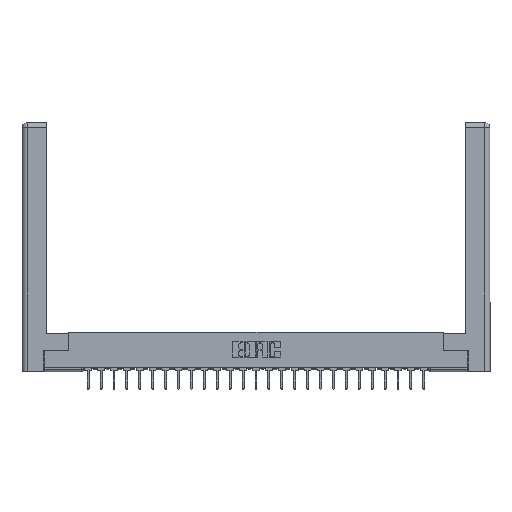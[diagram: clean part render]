
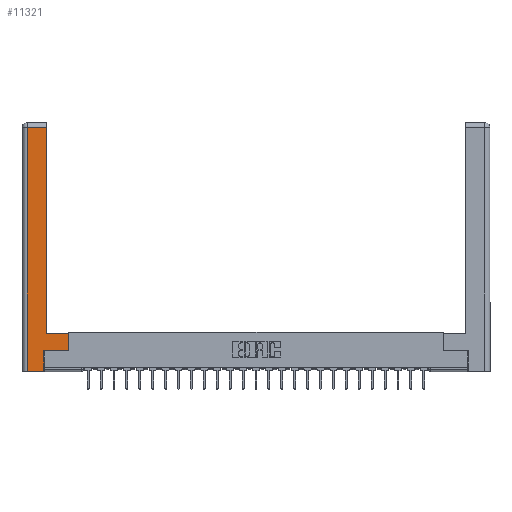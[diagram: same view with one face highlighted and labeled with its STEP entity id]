
A CAD part, top view. The second image highlights one B-rep face of the part: STEP entity #11321.
In plain terms, the highlighted planar face has unit normal (0, 0, 1).
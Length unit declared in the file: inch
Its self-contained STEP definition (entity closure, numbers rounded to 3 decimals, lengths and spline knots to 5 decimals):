
#91 = DIRECTION ( 'NONE',  ( 0., 1., 0. ) ) ;
#453 = VERTEX_POINT ( 'NONE', #3930 ) ;
#1445 = DIRECTION ( 'NONE',  ( 0., -1., 0. ) ) ;
#2126 = LINE ( 'NONE', #8370, #24151 ) ;
#2613 = VERTEX_POINT ( 'NONE', #10627 ) ;
#3254 = LINE ( 'NONE', #16500, #15256 ) ;
#3927 = LINE ( 'NONE', #7426, #9118 ) ;
#3930 = CARTESIAN_POINT ( 'NONE',  ( 0.565, 0.45, 0. ) ) ;
#4493 = VECTOR ( 'NONE', #9994, 39.37008 ) ;
#4917 = VERTEX_POINT ( 'NONE', #18198 ) ;
#4936 = FACE_OUTER_BOUND ( 'NONE', #17056, .T. ) ;
#4979 = VECTOR ( 'NONE', #1445, 39.37008 ) ;
#6336 = DIRECTION ( 'NONE',  ( 0., 1., 0. ) ) ;
#7166 = ORIENTED_EDGE ( 'NONE', *, *, #22486, .T. ) ;
#7337 = CARTESIAN_POINT ( 'NONE',  ( 0.295, 0.45, 0. ) ) ;
#7426 = CARTESIAN_POINT ( 'NONE',  ( 0.565, 0.45, 0. ) ) ;
#7503 = VERTEX_POINT ( 'NONE', #7896 ) ;
#7896 = CARTESIAN_POINT ( 'NONE',  ( 0.265, 0.245, 0. ) ) ;
#8370 = CARTESIAN_POINT ( 'NONE',  ( 0.265, 0.245, 0. ) ) ;
#8605 = VERTEX_POINT ( 'NONE', #7337 ) ;
#9118 = VECTOR ( 'NONE', #16224, 39.37008 ) ;
#9213 = CARTESIAN_POINT ( 'NONE',  ( 0.0615, 2.94, 0. ) ) ;
#9342 = LINE ( 'NONE', #14629, #14463 ) ;
#9994 = DIRECTION ( 'NONE',  ( -1., 0., 0. ) ) ;
#10014 = DIRECTION ( 'NONE',  ( 1., 0., 0. ) ) ;
#10089 = AXIS2_PLACEMENT_3D ( 'NONE', #15888, #20520, #24649 ) ;
#10627 = CARTESIAN_POINT ( 'NONE',  ( 0.565, 0.245, 0. ) ) ;
#10647 = EDGE_CURVE ( 'NONE', #2613, #453, #3927, .T. ) ;
#10920 = VERTEX_POINT ( 'NONE', #11051 ) ;
#11051 = CARTESIAN_POINT ( 'NONE',  ( 0.265, 0., 0. ) ) ;
#11321 = ADVANCED_FACE ( 'NONE', ( #4936 ), #16072, .F. ) ;
#12737 = LINE ( 'NONE', #27295, #4493 ) ;
#13498 = DIRECTION ( 'NONE',  ( -1., 0., 0. ) ) ;
#14463 = VECTOR ( 'NONE', #91, 39.37008 ) ;
#14501 = CARTESIAN_POINT ( 'NONE',  ( 0.0615, 0., 0. ) ) ;
#14629 = CARTESIAN_POINT ( 'NONE',  ( 0.295, 3., 0. ) ) ;
#14722 = EDGE_CURVE ( 'NONE', #7503, #2613, #15604, .T. ) ;
#15256 = VECTOR ( 'NONE', #10014, 39.37008 ) ;
#15604 = LINE ( 'NONE', #20770, #19044 ) ;
#15867 = CARTESIAN_POINT ( 'NONE',  ( 0.0615, 2.94, 0. ) ) ;
#15888 = CARTESIAN_POINT ( 'NONE',  ( 0., 0., 0. ) ) ;
#16072 = PLANE ( 'NONE',  #10089 ) ;
#16224 = DIRECTION ( 'NONE',  ( 0., 1., 0. ) ) ;
#16500 = CARTESIAN_POINT ( 'NONE',  ( 0.265, 0., 0. ) ) ;
#16535 = ORIENTED_EDGE ( 'NONE', *, *, #26457, .T. ) ;
#17056 = EDGE_LOOP ( 'NONE', ( #26391, #23812, #16535, #21348, #7166, #18307, #26395, #25398 ) ) ;
#18198 = CARTESIAN_POINT ( 'NONE',  ( 0.295, 2.94, 0. ) ) ;
#18307 = ORIENTED_EDGE ( 'NONE', *, *, #14722, .T. ) ;
#18453 = EDGE_CURVE ( 'NONE', #4917, #27498, #20606, .T. ) ;
#18882 = VECTOR ( 'NONE', #13498, 39.37008 ) ;
#19044 = VECTOR ( 'NONE', #24805, 39.37008 ) ;
#19745 = LINE ( 'NONE', #14501, #4979 ) ;
#20520 = DIRECTION ( 'NONE',  ( 0., 0., -1. ) ) ;
#20606 = LINE ( 'NONE', #15867, #18882 ) ;
#20770 = CARTESIAN_POINT ( 'NONE',  ( 0.565, 0.245, 0. ) ) ;
#21348 = ORIENTED_EDGE ( 'NONE', *, *, #26438, .T. ) ;
#22486 = EDGE_CURVE ( 'NONE', #10920, #7503, #2126, .T. ) ;
#23812 = ORIENTED_EDGE ( 'NONE', *, *, #18453, .T. ) ;
#24136 = EDGE_CURVE ( 'NONE', #453, #8605, #12737, .T. ) ;
#24144 = VERTEX_POINT ( 'NONE', #27565 ) ;
#24151 = VECTOR ( 'NONE', #6336, 39.37008 ) ;
#24649 = DIRECTION ( 'NONE',  ( -1., 0., 0. ) ) ;
#24805 = DIRECTION ( 'NONE',  ( 1., 0., 0. ) ) ;
#25398 = ORIENTED_EDGE ( 'NONE', *, *, #24136, .T. ) ;
#26391 = ORIENTED_EDGE ( 'NONE', *, *, #28307, .T. ) ;
#26395 = ORIENTED_EDGE ( 'NONE', *, *, #10647, .T. ) ;
#26438 = EDGE_CURVE ( 'NONE', #24144, #10920, #3254, .T. ) ;
#26457 = EDGE_CURVE ( 'NONE', #27498, #24144, #19745, .T. ) ;
#27295 = CARTESIAN_POINT ( 'NONE',  ( 0.295, 0.45, 0. ) ) ;
#27498 = VERTEX_POINT ( 'NONE', #9213 ) ;
#27565 = CARTESIAN_POINT ( 'NONE',  ( 0.0615, 0., 0. ) ) ;
#28307 = EDGE_CURVE ( 'NONE', #8605, #4917, #9342, .T. ) ;
